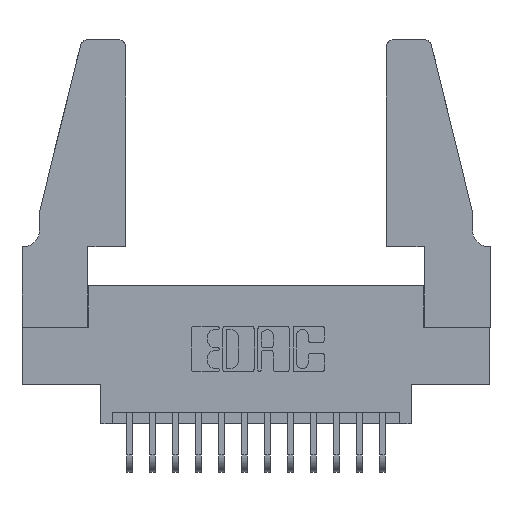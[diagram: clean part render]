
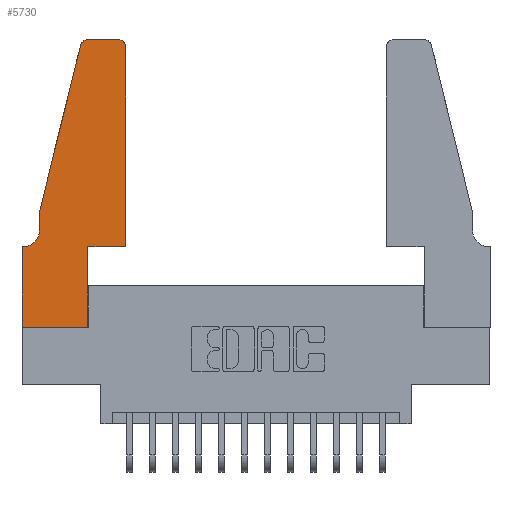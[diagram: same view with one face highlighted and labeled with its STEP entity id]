
A CAD part, top view. The second image highlights one B-rep face of the part: STEP entity #5730.
In plain terms, the highlighted planar face has unit normal (0, 0, 1).
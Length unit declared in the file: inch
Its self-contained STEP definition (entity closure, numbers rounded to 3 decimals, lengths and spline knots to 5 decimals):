
#74 = CARTESIAN_POINT ( 'NONE',  ( 0., 0.35, 0.37 ) ) ;
#237 = CARTESIAN_POINT ( 'NONE',  ( 0.0755, 0.35, 0.37 ) ) ;
#346 = DIRECTION ( 'NONE',  ( 0., 0., 1. ) ) ;
#564 = VECTOR ( 'NONE', #8327, 39.37008 ) ;
#646 = LINE ( 'NONE', #11041, #15991 ) ;
#738 = DIRECTION ( 'NONE',  ( 1., 0., 0. ) ) ;
#920 = CIRCLE ( 'NONE', #4407, 0.03 ) ;
#983 = LINE ( 'NONE', #16514, #564 ) ;
#994 = ORIENTED_EDGE ( 'NONE', *, *, #8981, .T. ) ;
#1062 = VERTEX_POINT ( 'NONE', #16724 ) ;
#1099 = EDGE_CURVE ( 'NONE', #9456, #4513, #6086, .T. ) ;
#1591 = DIRECTION ( 'NONE',  ( -1., 0., 0. ) ) ;
#1600 = VECTOR ( 'NONE', #15319, 39.37008 ) ;
#1691 = CARTESIAN_POINT ( 'NONE',  ( 0.4205, 1.22, 0.37 ) ) ;
#1727 = CARTESIAN_POINT ( 'NONE',  ( 0., 0.35, 0.37 ) ) ;
#1773 = EDGE_CURVE ( 'NONE', #1062, #7243, #7988, .T. ) ;
#1808 = ORIENTED_EDGE ( 'NONE', *, *, #1773, .T. ) ;
#2499 = VECTOR ( 'NONE', #5898, 39.37008 ) ;
#2551 = DIRECTION ( 'NONE',  ( -0.239, -0.971, 0. ) ) ;
#2596 = DIRECTION ( 'NONE',  ( -1., 0., 0. ) ) ;
#3035 = EDGE_CURVE ( 'NONE', #3602, #13937, #7326, .T. ) ;
#3212 = DIRECTION ( 'NONE',  ( 1., 0., 0. ) ) ;
#3341 = ORIENTED_EDGE ( 'NONE', *, *, #16311, .T. ) ;
#3602 = VERTEX_POINT ( 'NONE', #12387 ) ;
#3615 = EDGE_CURVE ( 'NONE', #4587, #12555, #8995, .T. ) ;
#3759 = EDGE_LOOP ( 'NONE', ( #994, #3341, #15312, #15665, #14616, #7448, #5426, #3841, #1808, #5008, #16251, #17253 ) ) ;
#3769 = CARTESIAN_POINT ( 'NONE',  ( 0., 0., 0.37 ) ) ;
#3841 = ORIENTED_EDGE ( 'NONE', *, *, #4866, .T. ) ;
#3925 = LINE ( 'NONE', #11874, #12563 ) ;
#4360 = LINE ( 'NONE', #3769, #16780 ) ;
#4366 = CARTESIAN_POINT ( 'NONE',  ( 0.25487, 1.22718, 0.37 ) ) ;
#4407 = AXIS2_PLACEMENT_3D ( 'NONE', #15240, #346, #3212 ) ;
#4513 = VERTEX_POINT ( 'NONE', #8114 ) ;
#4587 = VERTEX_POINT ( 'NONE', #12088 ) ;
#4866 = EDGE_CURVE ( 'NONE', #5647, #1062, #983, .T. ) ;
#4948 = CARTESIAN_POINT ( 'NONE',  ( 0.2865, 0.35, 0.37 ) ) ;
#5008 = ORIENTED_EDGE ( 'NONE', *, *, #11884, .T. ) ;
#5022 = VERTEX_POINT ( 'NONE', #14383 ) ;
#5109 = DIRECTION ( 'NONE',  ( 0., -1., 0. ) ) ;
#5342 = VECTOR ( 'NONE', #1591, 39.37008 ) ;
#5426 = ORIENTED_EDGE ( 'NONE', *, *, #5536, .T. ) ;
#5536 = EDGE_CURVE ( 'NONE', #12555, #5647, #4360, .T. ) ;
#5647 = VERTEX_POINT ( 'NONE', #11987 ) ;
#5730 = ADVANCED_FACE ( 'NONE', ( #7127 ), #10995, .T. ) ;
#5862 = CARTESIAN_POINT ( 'NONE',  ( 0.2865, 0.35, 0.37 ) ) ;
#5898 = DIRECTION ( 'NONE',  ( 0., 1., 0. ) ) ;
#6086 = LINE ( 'NONE', #14022, #2499 ) ;
#6341 = DIRECTION ( 'NONE',  ( 0., -1., 0. ) ) ;
#6453 = VERTEX_POINT ( 'NONE', #16301 ) ;
#6590 = VECTOR ( 'NONE', #738, 39.37008 ) ;
#6813 = CIRCLE ( 'NONE', #16014, 0.07 ) ;
#7127 = FACE_OUTER_BOUND ( 'NONE', #3759, .T. ) ;
#7243 = VERTEX_POINT ( 'NONE', #4948 ) ;
#7322 = CARTESIAN_POINT ( 'NONE',  ( 0.4505, 0.35, 0.37 ) ) ;
#7326 = LINE ( 'NONE', #15687, #10652 ) ;
#7448 = ORIENTED_EDGE ( 'NONE', *, *, #3615, .T. ) ;
#7903 = CARTESIAN_POINT ( 'NONE',  ( 0.0755, 0.42, 0.37 ) ) ;
#7988 = LINE ( 'NONE', #5862, #1600 ) ;
#8097 = DIRECTION ( 'NONE',  ( 0., 0., -1. ) ) ;
#8114 = CARTESIAN_POINT ( 'NONE',  ( 0.4505, 1.22, 0.37 ) ) ;
#8313 = LINE ( 'NONE', #7322, #6590 ) ;
#8327 = DIRECTION ( 'NONE',  ( 1., 0., 0. ) ) ;
#8981 = EDGE_CURVE ( 'NONE', #6453, #5022, #646, .T. ) ;
#8995 = LINE ( 'NONE', #237, #5342 ) ;
#9456 = VERTEX_POINT ( 'NONE', #16830 ) ;
#9667 = DIRECTION ( 'NONE',  ( 1., 0., 0. ) ) ;
#10652 = VECTOR ( 'NONE', #6341, 39.37008 ) ;
#10729 = CARTESIAN_POINT ( 'NONE',  ( 0.0055, 0.42, 0.37 ) ) ;
#10877 = EDGE_CURVE ( 'NONE', #13937, #4587, #6813, .T. ) ;
#10880 = DIRECTION ( 'NONE',  ( 0., 0., 1. ) ) ;
#10995 = PLANE ( 'NONE',  #16868 ) ;
#11041 = CARTESIAN_POINT ( 'NONE',  ( 0.2605, 1.25, 0.37 ) ) ;
#11370 = CIRCLE ( 'NONE', #14627, 0.03 ) ;
#11874 = CARTESIAN_POINT ( 'NONE',  ( 0.0755, 0.5, 0.37 ) ) ;
#11884 = EDGE_CURVE ( 'NONE', #7243, #9456, #8313, .T. ) ;
#11987 = CARTESIAN_POINT ( 'NONE',  ( 0., 0., 0.37 ) ) ;
#12088 = CARTESIAN_POINT ( 'NONE',  ( 0.0055, 0.35, 0.37 ) ) ;
#12387 = CARTESIAN_POINT ( 'NONE',  ( 0.0755, 0.5, 0.37 ) ) ;
#12555 = VERTEX_POINT ( 'NONE', #1727 ) ;
#12563 = VECTOR ( 'NONE', #2551, 39.37008 ) ;
#13656 = DIRECTION ( 'NONE',  ( 0., 0., 1. ) ) ;
#13937 = VERTEX_POINT ( 'NONE', #7903 ) ;
#14022 = CARTESIAN_POINT ( 'NONE',  ( 0.4505, 0.35, 0.37 ) ) ;
#14068 = VERTEX_POINT ( 'NONE', #4366 ) ;
#14383 = CARTESIAN_POINT ( 'NONE',  ( 0.284, 1.25, 0.37 ) ) ;
#14421 = EDGE_CURVE ( 'NONE', #4513, #6453, #11370, .T. ) ;
#14616 = ORIENTED_EDGE ( 'NONE', *, *, #10877, .T. ) ;
#14627 = AXIS2_PLACEMENT_3D ( 'NONE', #1691, #13656, #15110 ) ;
#15059 = DIRECTION ( 'NONE',  ( -1., 0., 0. ) ) ;
#15110 = DIRECTION ( 'NONE',  ( 1., 0., 0. ) ) ;
#15240 = CARTESIAN_POINT ( 'NONE',  ( 0.284, 1.22, 0.37 ) ) ;
#15312 = ORIENTED_EDGE ( 'NONE', *, *, #15517, .T. ) ;
#15319 = DIRECTION ( 'NONE',  ( 0., 1., 0. ) ) ;
#15517 = EDGE_CURVE ( 'NONE', #14068, #3602, #3925, .T. ) ;
#15665 = ORIENTED_EDGE ( 'NONE', *, *, #3035, .T. ) ;
#15687 = CARTESIAN_POINT ( 'NONE',  ( 0.0755, 0.5, 0.37 ) ) ;
#15991 = VECTOR ( 'NONE', #15059, 39.37008 ) ;
#16014 = AXIS2_PLACEMENT_3D ( 'NONE', #10729, #8097, #2596 ) ;
#16251 = ORIENTED_EDGE ( 'NONE', *, *, #1099, .T. ) ;
#16301 = CARTESIAN_POINT ( 'NONE',  ( 0.4205, 1.25, 0.37 ) ) ;
#16311 = EDGE_CURVE ( 'NONE', #5022, #14068, #920, .T. ) ;
#16514 = CARTESIAN_POINT ( 'NONE',  ( 0., 0., 0.37 ) ) ;
#16724 = CARTESIAN_POINT ( 'NONE',  ( 0.2865, 0., 0.37 ) ) ;
#16780 = VECTOR ( 'NONE', #5109, 39.37008 ) ;
#16830 = CARTESIAN_POINT ( 'NONE',  ( 0.4505, 0.35, 0.37 ) ) ;
#16868 = AXIS2_PLACEMENT_3D ( 'NONE', #74, #10880, #9667 ) ;
#17253 = ORIENTED_EDGE ( 'NONE', *, *, #14421, .T. ) ;
